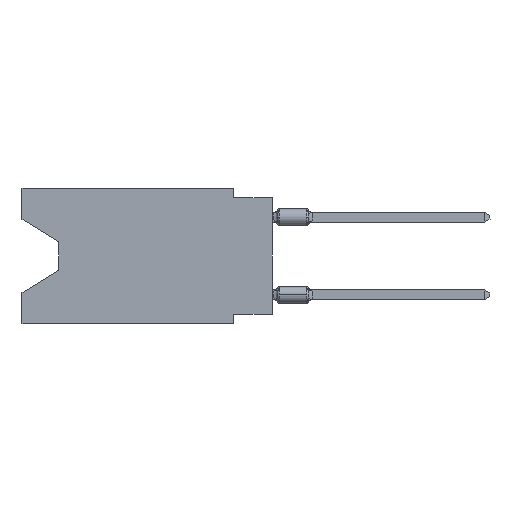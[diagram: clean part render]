
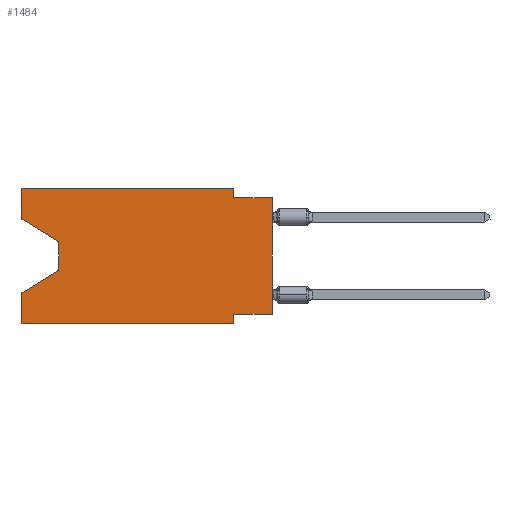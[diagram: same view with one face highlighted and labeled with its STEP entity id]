
A CAD part, left-side view. The second image highlights one B-rep face of the part: STEP entity #1484.
In plain terms, the highlighted planar face has unit normal (-1, 0, 0).
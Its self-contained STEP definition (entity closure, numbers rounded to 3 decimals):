
#108 = CARTESIAN_POINT ( 'NONE',  ( 0., 0., -0.635 ) ) ;
#110 = VECTOR ( 'NONE', #5463, 1000. ) ;
#174 = EDGE_CURVE ( 'NONE', #5097, #4951, #12241, .T. ) ;
#214 = EDGE_CURVE ( 'NONE', #10266, #19766, #10503, .T. ) ;
#226 = EDGE_CURVE ( 'NONE', #20998, #19766, #16155, .T. ) ;
#257 = DIRECTION ( 'NONE',  ( 0., 0., -1. ) ) ;
#1072 = CARTESIAN_POINT ( 'NONE',  ( 0., 13.97, -3.505 ) ) ;
#1231 = ORIENTED_EDGE ( 'NONE', *, *, #8698, .F. ) ;
#1324 = VERTEX_POINT ( 'NONE', #8445 ) ;
#1484 = ADVANCED_FACE ( 'NONE', ( #17656 ), #1997, .F. ) ;
#1876 = CARTESIAN_POINT ( 'NONE',  ( 0., 16.383, 0. ) ) ;
#1934 = CARTESIAN_POINT ( 'NONE',  ( 0., 0., -0.635 ) ) ;
#1997 = PLANE ( 'NONE',  #8204 ) ;
#2143 = LINE ( 'NONE', #10883, #6829 ) ;
#2332 = DIRECTION ( 'NONE',  ( 0., 0., 1. ) ) ;
#2720 = VECTOR ( 'NONE', #2332, 1000. ) ;
#2779 = CARTESIAN_POINT ( 'NONE',  ( 0., 0., 0. ) ) ;
#2834 = ORIENTED_EDGE ( 'NONE', *, *, #10091, .F. ) ;
#3171 = DIRECTION ( 'NONE',  ( 0., 0., -1. ) ) ;
#3623 = ORIENTED_EDGE ( 'NONE', *, *, #7905, .T. ) ;
#3656 = DIRECTION ( 'NONE',  ( 0., -1., 0. ) ) ;
#3716 = VECTOR ( 'NONE', #5557, 1000. ) ;
#3957 = CARTESIAN_POINT ( 'NONE',  ( 0., 13.97, -3.505 ) ) ;
#4526 = ORIENTED_EDGE ( 'NONE', *, *, #22288, .T. ) ;
#4631 = LINE ( 'NONE', #20836, #12507 ) ;
#4951 = VERTEX_POINT ( 'NONE', #11925 ) ;
#5096 = DIRECTION ( 'NONE',  ( 0., 0.855, -0.519 ) ) ;
#5097 = VERTEX_POINT ( 'NONE', #17895 ) ;
#5441 = DIRECTION ( 'NONE',  ( 0., 0., 1. ) ) ;
#5463 = DIRECTION ( 'NONE',  ( 0., 0., -1. ) ) ;
#5557 = DIRECTION ( 'NONE',  ( 0., 1., 0. ) ) ;
#5609 = ORIENTED_EDGE ( 'NONE', *, *, #18879, .F. ) ;
#5944 = CARTESIAN_POINT ( 'NONE',  ( 0., 2.54, 0. ) ) ;
#6491 = DIRECTION ( 'NONE',  ( 0., 0., -1. ) ) ;
#6829 = VECTOR ( 'NONE', #21154, 1000. ) ;
#6910 = EDGE_CURVE ( 'NONE', #20922, #22287, #9176, .T. ) ;
#6936 = CARTESIAN_POINT ( 'NONE',  ( 0., 0., -8.255 ) ) ;
#7743 = LINE ( 'NONE', #10039, #18642 ) ;
#7905 = EDGE_CURVE ( 'NONE', #5097, #22287, #9576, .T. ) ;
#8089 = EDGE_LOOP ( 'NONE', ( #17809, #9853, #22729, #16687, #4526, #2834, #20542, #3623, #18143, #5609, #1231, #10675 ) ) ;
#8204 = AXIS2_PLACEMENT_3D ( 'NONE', #9011, #17880, #257 ) ;
#8407 = VECTOR ( 'NONE', #9834, 1000. ) ;
#8445 = CARTESIAN_POINT ( 'NONE',  ( 0., 16.383, -2.038 ) ) ;
#8698 = EDGE_CURVE ( 'NONE', #22304, #21703, #14584, .T. ) ;
#8859 = VECTOR ( 'NONE', #5441, 1000. ) ;
#9011 = CARTESIAN_POINT ( 'NONE',  ( 0., 16.383, 0. ) ) ;
#9063 = VECTOR ( 'NONE', #6491, 1000. ) ;
#9176 = LINE ( 'NONE', #1934, #18606 ) ;
#9261 = VERTEX_POINT ( 'NONE', #11769 ) ;
#9576 = LINE ( 'NONE', #2779, #2720 ) ;
#9834 = DIRECTION ( 'NONE',  ( 0., -1., 0. ) ) ;
#9853 = ORIENTED_EDGE ( 'NONE', *, *, #13583, .T. ) ;
#10039 = CARTESIAN_POINT ( 'NONE',  ( 0., 16.383, 0. ) ) ;
#10091 = EDGE_CURVE ( 'NONE', #4951, #9261, #22099, .T. ) ;
#10266 = VERTEX_POINT ( 'NONE', #11116 ) ;
#10503 = LINE ( 'NONE', #1876, #8859 ) ;
#10675 = ORIENTED_EDGE ( 'NONE', *, *, #19349, .F. ) ;
#10883 = CARTESIAN_POINT ( 'NONE',  ( 0., 16.383, -2.038 ) ) ;
#11116 = CARTESIAN_POINT ( 'NONE',  ( 0., 16.383, -8.89 ) ) ;
#11569 = CARTESIAN_POINT ( 'NONE',  ( 0., 16.383, 0. ) ) ;
#11657 = DIRECTION ( 'NONE',  ( 0., 0., 1. ) ) ;
#11769 = CARTESIAN_POINT ( 'NONE',  ( 0., 2.54, -8.89 ) ) ;
#11925 = CARTESIAN_POINT ( 'NONE',  ( 0., 2.54, -8.255 ) ) ;
#12241 = LINE ( 'NONE', #6936, #3716 ) ;
#12507 = VECTOR ( 'NONE', #21079, 1000. ) ;
#13355 = CARTESIAN_POINT ( 'NONE',  ( 0., 13.97, -5.385 ) ) ;
#13583 = EDGE_CURVE ( 'NONE', #13726, #20998, #21584, .T. ) ;
#13726 = VERTEX_POINT ( 'NONE', #1072 ) ;
#13922 = CARTESIAN_POINT ( 'NONE',  ( 0., 16.383, 0. ) ) ;
#14413 = CARTESIAN_POINT ( 'NONE',  ( 0., 13.97, -5.385 ) ) ;
#14584 = LINE ( 'NONE', #11569, #8407 ) ;
#16155 = LINE ( 'NONE', #14413, #18798 ) ;
#16687 = ORIENTED_EDGE ( 'NONE', *, *, #214, .F. ) ;
#16751 = LINE ( 'NONE', #22285, #9063 ) ;
#17656 = FACE_OUTER_BOUND ( 'NONE', #8089, .T. ) ;
#17809 = ORIENTED_EDGE ( 'NONE', *, *, #21628, .T. ) ;
#17880 = DIRECTION ( 'NONE',  ( 1., 0., 0. ) ) ;
#17895 = CARTESIAN_POINT ( 'NONE',  ( 0., 0., -8.255 ) ) ;
#18143 = ORIENTED_EDGE ( 'NONE', *, *, #6910, .F. ) ;
#18606 = VECTOR ( 'NONE', #3656, 1000. ) ;
#18642 = VECTOR ( 'NONE', #11657, 1000. ) ;
#18798 = VECTOR ( 'NONE', #5096, 1000. ) ;
#18879 = EDGE_CURVE ( 'NONE', #21703, #20922, #16751, .T. ) ;
#18956 = CARTESIAN_POINT ( 'NONE',  ( 0., 2.54, -8.89 ) ) ;
#19349 = EDGE_CURVE ( 'NONE', #1324, #22304, #7743, .T. ) ;
#19766 = VERTEX_POINT ( 'NONE', #22126 ) ;
#20542 = ORIENTED_EDGE ( 'NONE', *, *, #174, .F. ) ;
#20836 = CARTESIAN_POINT ( 'NONE',  ( 0., 16.383, -8.89 ) ) ;
#20922 = VERTEX_POINT ( 'NONE', #21444 ) ;
#20941 = VECTOR ( 'NONE', #3171, 1000. ) ;
#20998 = VERTEX_POINT ( 'NONE', #13355 ) ;
#21079 = DIRECTION ( 'NONE',  ( 0., -1., 0. ) ) ;
#21154 = DIRECTION ( 'NONE',  ( 0., -0.855, -0.519 ) ) ;
#21444 = CARTESIAN_POINT ( 'NONE',  ( 0., 2.54, -0.635 ) ) ;
#21584 = LINE ( 'NONE', #3957, #110 ) ;
#21628 = EDGE_CURVE ( 'NONE', #1324, #13726, #2143, .T. ) ;
#21703 = VERTEX_POINT ( 'NONE', #5944 ) ;
#22099 = LINE ( 'NONE', #18956, #20941 ) ;
#22126 = CARTESIAN_POINT ( 'NONE',  ( 0., 16.383, -6.852 ) ) ;
#22285 = CARTESIAN_POINT ( 'NONE',  ( 0., 2.54, 0. ) ) ;
#22287 = VERTEX_POINT ( 'NONE', #108 ) ;
#22288 = EDGE_CURVE ( 'NONE', #10266, #9261, #4631, .T. ) ;
#22304 = VERTEX_POINT ( 'NONE', #13922 ) ;
#22729 = ORIENTED_EDGE ( 'NONE', *, *, #226, .T. ) ;
